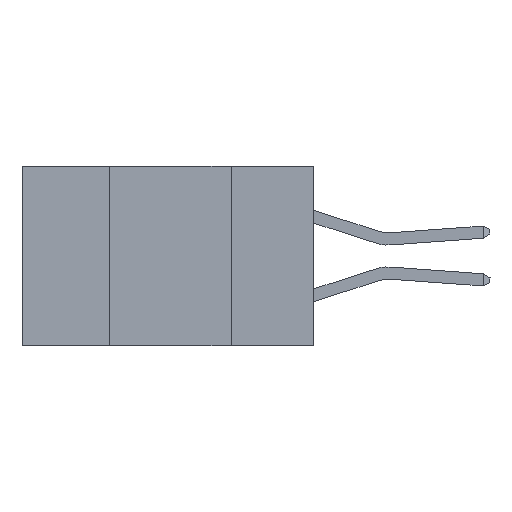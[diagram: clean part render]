
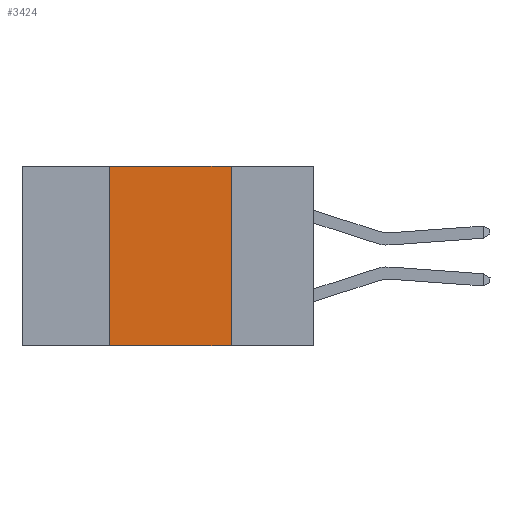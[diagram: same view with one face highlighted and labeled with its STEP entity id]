
A CAD part, left-side view. The second image highlights one B-rep face of the part: STEP entity #3424.
In plain terms, the highlighted planar face has unit normal (-1, 0, 0).
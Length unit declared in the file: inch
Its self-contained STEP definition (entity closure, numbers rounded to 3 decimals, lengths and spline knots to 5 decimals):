
#2225 = DIRECTION ( 'NONE',  ( 1., 0., 0. ) ) ;
#3424 = ADVANCED_FACE ( 'NONE', ( #39791 ), #10607, .F. ) ;
#4219 = VECTOR ( 'NONE', #6361, 39.37008 ) ;
#4742 = LINE ( 'NONE', #30952, #5186 ) ;
#5186 = VECTOR ( 'NONE', #17730, 39.37008 ) ;
#6361 = DIRECTION ( 'NONE',  ( 0., 0., -1. ) ) ;
#6653 = VECTOR ( 'NONE', #11098, 39.37008 ) ;
#7414 = DIRECTION ( 'NONE',  ( 0., 0., -1. ) ) ;
#9640 = EDGE_CURVE ( 'NONE', #37741, #31850, #35325, .T. ) ;
#10607 = PLANE ( 'NONE',  #39314 ) ;
#11098 = DIRECTION ( 'NONE',  ( 0., -1., 0. ) ) ;
#13843 = CARTESIAN_POINT ( 'NONE',  ( 0., 0.42, 0. ) ) ;
#14290 = LINE ( 'NONE', #27310, #6653 ) ;
#17730 = DIRECTION ( 'NONE',  ( 0., 0., 1. ) ) ;
#18363 = EDGE_LOOP ( 'NONE', ( #35450, #41048, #28451, #21579 ) ) ;
#19765 = CARTESIAN_POINT ( 'NONE',  ( 0., 0.17, 0. ) ) ;
#20453 = EDGE_CURVE ( 'NONE', #39644, #31850, #33607, .T. ) ;
#20829 = DIRECTION ( 'NONE',  ( 0., -1., 0. ) ) ;
#21550 = EDGE_CURVE ( 'NONE', #39644, #29109, #4742, .T. ) ;
#21579 = ORIENTED_EDGE ( 'NONE', *, *, #20453, .T. ) ;
#23426 = EDGE_CURVE ( 'NONE', #29109, #37741, #14290, .T. ) ;
#24016 = CARTESIAN_POINT ( 'NONE',  ( 0., 0.42, -0.37 ) ) ;
#27310 = CARTESIAN_POINT ( 'NONE',  ( 0., 0.6, 0. ) ) ;
#28451 = ORIENTED_EDGE ( 'NONE', *, *, #21550, .F. ) ;
#29109 = VERTEX_POINT ( 'NONE', #13843 ) ;
#29593 = VECTOR ( 'NONE', #20829, 39.37008 ) ;
#30042 = CARTESIAN_POINT ( 'NONE',  ( 0., 0.17, 0. ) ) ;
#30952 = CARTESIAN_POINT ( 'NONE',  ( 0., 0.42, 0. ) ) ;
#31850 = VERTEX_POINT ( 'NONE', #36063 ) ;
#33607 = LINE ( 'NONE', #36384, #29593 ) ;
#34597 = CARTESIAN_POINT ( 'NONE',  ( 0., 0.6, 0. ) ) ;
#35325 = LINE ( 'NONE', #19765, #4219 ) ;
#35450 = ORIENTED_EDGE ( 'NONE', *, *, #9640, .F. ) ;
#36063 = CARTESIAN_POINT ( 'NONE',  ( 0., 0.17, -0.37 ) ) ;
#36384 = CARTESIAN_POINT ( 'NONE',  ( 0., 0.6, -0.37 ) ) ;
#37741 = VERTEX_POINT ( 'NONE', #30042 ) ;
#39314 = AXIS2_PLACEMENT_3D ( 'NONE', #34597, #2225, #7414 ) ;
#39644 = VERTEX_POINT ( 'NONE', #24016 ) ;
#39791 = FACE_OUTER_BOUND ( 'NONE', #18363, .T. ) ;
#41048 = ORIENTED_EDGE ( 'NONE', *, *, #23426, .F. ) ;
